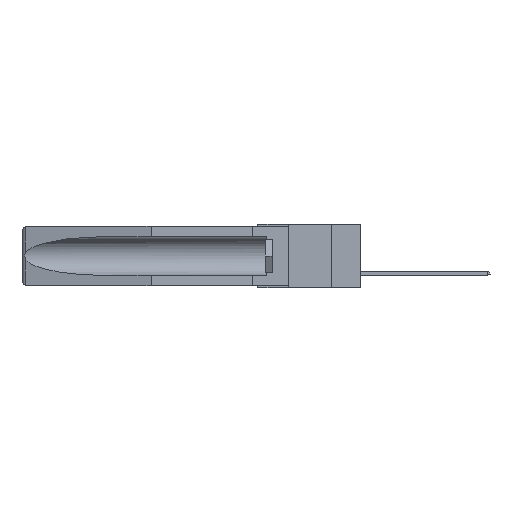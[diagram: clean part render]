
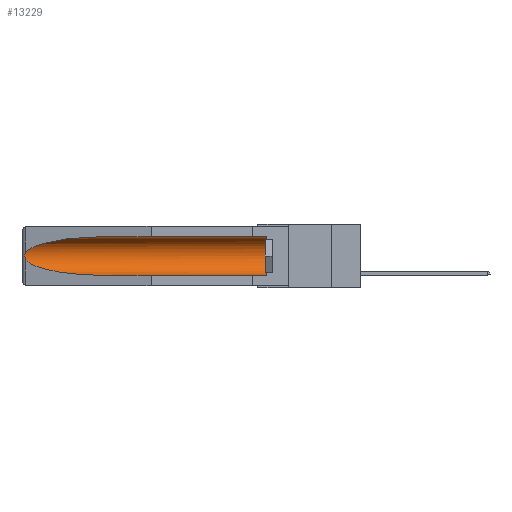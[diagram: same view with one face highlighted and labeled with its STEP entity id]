
A CAD part, left-side view. The second image highlights one B-rep face of the part: STEP entity #13229.
In plain terms, the highlighted cylindrical face has radius 2.857 mm (diameter 5.715 mm), a partial arc.
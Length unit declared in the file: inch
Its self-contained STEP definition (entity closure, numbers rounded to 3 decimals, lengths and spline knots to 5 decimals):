
#409 = CARTESIAN_POINT ( 'NONE',  ( 0.2673, 1.53269, -0.17917 ) ) ;
#666 = CARTESIAN_POINT ( 'NONE',  ( 0.26597, 1.5296, -0.19026 ) ) ;
#943 = CARTESIAN_POINT ( 'NONE',  ( 0.155, 1.07973, -0.059 ) ) ;
#963 = ORIENTED_EDGE ( 'NONE', *, *, #23032, .T. ) ;
#1043 = CARTESIAN_POINT ( 'NONE',  ( 0.155, 0.126, -0.284 ) ) ;
#1187 = B_SPLINE_CURVE_WITH_KNOTS ( 'NONE', 3,
 ( #23571, #23402, #2405, #25683, #8786, #25507, #409, #12998, #666, #23488 ),
 .UNSPECIFIED., .F., .F.,
 ( 4, 2, 2, 2, 4 ),
 ( 0., 0.00029, 0.00058, 0.00087, 0.00117 ),
 .UNSPECIFIED. ) ;
#1486 = CARTESIAN_POINT ( 'NONE',  ( 0.21114, 1.30732, -0.284 ) ) ;
#2405 = CARTESIAN_POINT ( 'NONE',  ( 0.26654, 1.53092, -0.15636 ) ) ;
#3300 = AXIS2_PLACEMENT_3D ( 'NONE', #21824, #25963, #23923 ) ;
#3377 = ORIENTED_EDGE ( 'NONE', *, *, #8931, .T. ) ;
#3544 = ORIENTED_EDGE ( 'NONE', *, *, #21414, .T. ) ;
#5399 = CARTESIAN_POINT ( 'NONE',  ( 0.155, 1.07973, -0.284 ) ) ;
#6898 = CARTESIAN_POINT ( 'NONE',  ( 0.25451, 1.48313, -0.09465 ) ) ;
#6922 = VECTOR ( 'NONE', #15591, 39.37008 ) ;
#7821 = DIRECTION ( 'NONE',  ( 0., 0., 1. ) ) ;
#8057 = ORIENTED_EDGE ( 'NONE', *, *, #26677, .T. ) ;
#8362 = FACE_OUTER_BOUND ( 'NONE', #25949, .T. ) ;
#8786 = CARTESIAN_POINT ( 'NONE',  ( 0.2675, 1.53308, -0.16763 ) ) ;
#8931 = EDGE_CURVE ( 'NONE', #24231, #19832, #20614, .T. ) ;
#9849 = LINE ( 'NONE', #22015, #6922 ) ;
#9927 = CIRCLE ( 'NONE', #3300, 0.1125 ) ;
#10322 = CYLINDRICAL_SURFACE ( 'NONE', #16297, 0.1125 ) ;
#11922 = VERTEX_POINT ( 'NONE', #22854 ) ;
#12557 = EDGE_CURVE ( 'NONE', #11922, #14088, #17734, .T. ) ;
#12998 = CARTESIAN_POINT ( 'NONE',  ( 0.26655, 1.53094, -0.18657 ) ) ;
#13196 = CARTESIAN_POINT ( 'NONE',  ( 0.21114, 1.30732, -0.059 ) ) ;
#13229 = ADVANCED_FACE ( 'NONE', ( #8362 ), #10322, .F. ) ;
#13394 = DIRECTION ( 'NONE',  ( 0., 1., 0. ) ) ;
#13689 = VERTEX_POINT ( 'NONE', #21605 ) ;
#14088 = VERTEX_POINT ( 'NONE', #23245 ) ;
#15591 = DIRECTION ( 'NONE',  ( 0., 1., 0. ) ) ;
#16297 = AXIS2_PLACEMENT_3D ( 'NONE', #23895, #13394, #7821 ) ;
#16741 = ORIENTED_EDGE ( 'NONE', *, *, #12557, .T. ) ;
#16970 = DIRECTION ( 'NONE',  ( 0., 1., 0. ) ) ;
#17704 = ORIENTED_EDGE ( 'NONE', *, *, #24869, .F. ) ;
#17734 =( BOUNDED_CURVE ( )  B_SPLINE_CURVE ( 3, ( #943, #13196, #6898, #25719 ),
 .UNSPECIFIED., .F., .F. ) 
 B_SPLINE_CURVE_WITH_KNOTS ( ( 4, 4 ),
 ( 4.71239, 6.08839 ),
 .UNSPECIFIED. ) 
 CURVE ( )  GEOMETRIC_REPRESENTATION_ITEM ( )  RATIONAL_B_SPLINE_CURVE ( ( 1., 0.848, 0.848, 1. ) ) 
 REPRESENTATION_ITEM ( '' )  );
#18175 = CARTESIAN_POINT ( 'NONE',  ( 0.25451, 1.48313, -0.24835 ) ) ;
#18436 = VERTEX_POINT ( 'NONE', #1043 ) ;
#19790 = LINE ( 'NONE', #21280, #21478 ) ;
#19832 = VERTEX_POINT ( 'NONE', #5399 ) ;
#20614 =( BOUNDED_CURVE ( )  B_SPLINE_CURVE ( 3, ( #22677, #18175, #1486, #24502 ),
 .UNSPECIFIED., .F., .F. ) 
 B_SPLINE_CURVE_WITH_KNOTS ( ( 4, 4 ),
 ( 0.1948, 1.5708 ),
 .UNSPECIFIED. ) 
 CURVE ( )  GEOMETRIC_REPRESENTATION_ITEM ( )  RATIONAL_B_SPLINE_CURVE ( ( 1., 0.848, 0.848, 1. ) ) 
 REPRESENTATION_ITEM ( '' )  );
#21280 = CARTESIAN_POINT ( 'NONE',  ( 0.155, -0.30754, -0.284 ) ) ;
#21414 = EDGE_CURVE ( 'NONE', #13689, #11922, #9849, .T. ) ;
#21478 = VECTOR ( 'NONE', #16970, 39.37008 ) ;
#21605 = CARTESIAN_POINT ( 'NONE',  ( 0.155, 0.126, -0.059 ) ) ;
#21824 = CARTESIAN_POINT ( 'NONE',  ( 0.155, 0.126, -0.1715 ) ) ;
#22015 = CARTESIAN_POINT ( 'NONE',  ( 0.155, -0.30754, -0.059 ) ) ;
#22677 = CARTESIAN_POINT ( 'NONE',  ( 0.26537, 1.52718, -0.19328 ) ) ;
#22854 = CARTESIAN_POINT ( 'NONE',  ( 0.155, 1.07973, -0.059 ) ) ;
#23032 = EDGE_CURVE ( 'NONE', #14088, #24231, #1187, .T. ) ;
#23245 = CARTESIAN_POINT ( 'NONE',  ( 0.26537, 1.52718, -0.14972 ) ) ;
#23402 = CARTESIAN_POINT ( 'NONE',  ( 0.26597, 1.52961, -0.15275 ) ) ;
#23488 = CARTESIAN_POINT ( 'NONE',  ( 0.26537, 1.52718, -0.19328 ) ) ;
#23571 = CARTESIAN_POINT ( 'NONE',  ( 0.26537, 1.52718, -0.14972 ) ) ;
#23895 = CARTESIAN_POINT ( 'NONE',  ( 0.155, -0.30754, -0.1715 ) ) ;
#23923 = DIRECTION ( 'NONE',  ( 0., 0., 1. ) ) ;
#24231 = VERTEX_POINT ( 'NONE', #26142 ) ;
#24502 = CARTESIAN_POINT ( 'NONE',  ( 0.155, 1.07973, -0.284 ) ) ;
#24869 = EDGE_CURVE ( 'NONE', #18436, #19832, #19790, .T. ) ;
#25507 = CARTESIAN_POINT ( 'NONE',  ( 0.2675, 1.53308, -0.17534 ) ) ;
#25683 = CARTESIAN_POINT ( 'NONE',  ( 0.2673, 1.5327, -0.16383 ) ) ;
#25719 = CARTESIAN_POINT ( 'NONE',  ( 0.26537, 1.52718, -0.14972 ) ) ;
#25949 = EDGE_LOOP ( 'NONE', ( #16741, #963, #3377, #17704, #8057, #3544 ) ) ;
#25963 = DIRECTION ( 'NONE',  ( 0., -1., 0. ) ) ;
#26142 = CARTESIAN_POINT ( 'NONE',  ( 0.26537, 1.52718, -0.19328 ) ) ;
#26677 = EDGE_CURVE ( 'NONE', #18436, #13689, #9927, .T. ) ;
